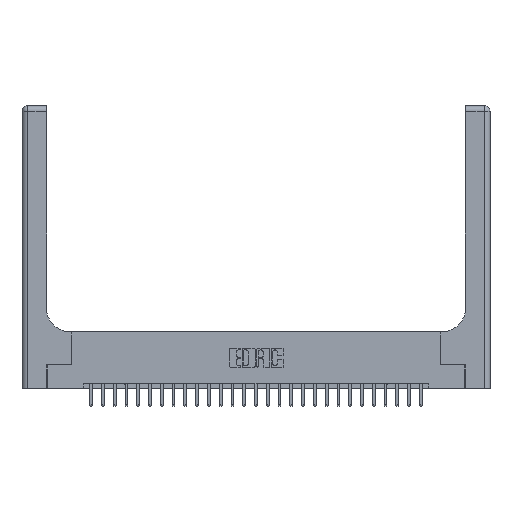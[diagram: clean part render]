
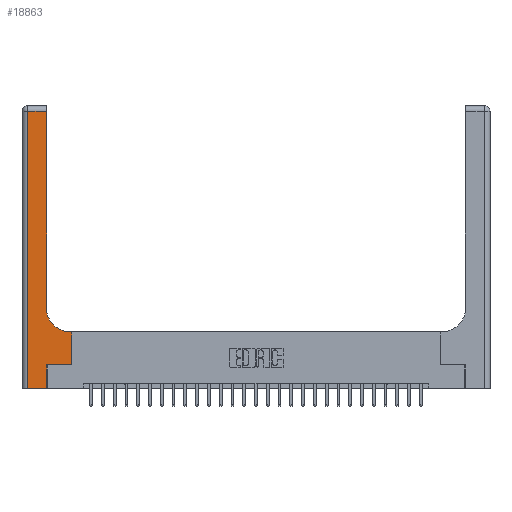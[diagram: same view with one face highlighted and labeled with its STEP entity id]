
A CAD part, top view. The second image highlights one B-rep face of the part: STEP entity #18863.
In plain terms, the highlighted planar face has unit normal (0, 0, 1).
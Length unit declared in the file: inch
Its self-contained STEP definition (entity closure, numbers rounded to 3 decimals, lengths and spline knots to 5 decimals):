
#50 = VERTEX_POINT ( 'NONE', #14233 ) ;
#340 = VERTEX_POINT ( 'NONE', #12329 ) ;
#403 = PLANE ( 'NONE',  #8619 ) ;
#505 = CARTESIAN_POINT ( 'NONE',  ( 0.51, 0.6, 0.37 ) ) ;
#557 = CARTESIAN_POINT ( 'NONE',  ( 0.528, 0.25, 0.37 ) ) ;
#688 = LINE ( 'NONE', #557, #17338 ) ;
#1341 = DIRECTION ( 'NONE',  ( 0., -1., 0. ) ) ;
#1430 = LINE ( 'NONE', #13756, #6898 ) ;
#2548 = DIRECTION ( 'NONE',  ( -1., 0., 0. ) ) ;
#2902 = ORIENTED_EDGE ( 'NONE', *, *, #24737, .T. ) ;
#2943 = EDGE_CURVE ( 'NONE', #15445, #6280, #25921, .T. ) ;
#3306 = EDGE_CURVE ( 'NONE', #50, #6949, #1430, .T. ) ;
#3812 = CARTESIAN_POINT ( 'NONE',  ( 0., 0., 0.37 ) ) ;
#3834 = VECTOR ( 'NONE', #21688, 39.37008 ) ;
#4189 = DIRECTION ( 'NONE',  ( 1., 0., 0. ) ) ;
#4561 = CARTESIAN_POINT ( 'NONE',  ( 0.265, 0.25, 0.37 ) ) ;
#4729 = CARTESIAN_POINT ( 'NONE',  ( 0.528, 0.25, 0.37 ) ) ;
#5106 = EDGE_CURVE ( 'NONE', #21176, #15445, #7725, .T. ) ;
#6278 = DIRECTION ( 'NONE',  ( 0., 0., -1. ) ) ;
#6280 = VERTEX_POINT ( 'NONE', #11537 ) ;
#6291 = CIRCLE ( 'NONE', #9298, 0.25 ) ;
#6699 = ORIENTED_EDGE ( 'NONE', *, *, #5106, .T. ) ;
#6898 = VECTOR ( 'NONE', #7549, 39.37008 ) ;
#6949 = VERTEX_POINT ( 'NONE', #505 ) ;
#7365 = CARTESIAN_POINT ( 'NONE',  ( 0.265, 0., 0.37 ) ) ;
#7463 = CARTESIAN_POINT ( 'NONE',  ( 0., 2.94, 0.37 ) ) ;
#7501 = EDGE_CURVE ( 'NONE', #340, #9209, #17818, .T. ) ;
#7549 = DIRECTION ( 'NONE',  ( -1., 0., 0. ) ) ;
#7725 = LINE ( 'NONE', #19927, #19897 ) ;
#7945 = ORIENTED_EDGE ( 'NONE', *, *, #13240, .T. ) ;
#8368 = ORIENTED_EDGE ( 'NONE', *, *, #14113, .T. ) ;
#8572 = CARTESIAN_POINT ( 'NONE',  ( 0., 3., 0.37 ) ) ;
#8619 = AXIS2_PLACEMENT_3D ( 'NONE', #8572, #6278, #2548 ) ;
#8847 = VECTOR ( 'NONE', #1341, 39.37008 ) ;
#9209 = VERTEX_POINT ( 'NONE', #4561 ) ;
#9298 = AXIS2_PLACEMENT_3D ( 'NONE', #22425, #16543, #4189 ) ;
#9631 = EDGE_LOOP ( 'NONE', ( #6699, #22606, #20917, #18238, #24569, #7945, #2902, #23261, #8368 ) ) ;
#9702 = DIRECTION ( 'NONE',  ( 1., 0., 0. ) ) ;
#9723 = EDGE_CURVE ( 'NONE', #6280, #15460, #14806, .T. ) ;
#10601 = DIRECTION ( 'NONE',  ( 0., 1., 0. ) ) ;
#11537 = CARTESIAN_POINT ( 'NONE',  ( 0.06, 2.94, 0.37 ) ) ;
#11619 = VECTOR ( 'NONE', #19183, 39.37008 ) ;
#12329 = CARTESIAN_POINT ( 'NONE',  ( 0.265, 0., 0.37 ) ) ;
#12386 = VERTEX_POINT ( 'NONE', #4729 ) ;
#13240 = EDGE_CURVE ( 'NONE', #9209, #12386, #19283, .T. ) ;
#13669 = CARTESIAN_POINT ( 'NONE',  ( 0.06, 3., 0.37 ) ) ;
#13756 = CARTESIAN_POINT ( 'NONE',  ( 0.26, 0.6, 0.37 ) ) ;
#14113 = EDGE_CURVE ( 'NONE', #6949, #21176, #6291, .T. ) ;
#14233 = CARTESIAN_POINT ( 'NONE',  ( 0.528, 0.6, 0.37 ) ) ;
#14250 = CARTESIAN_POINT ( 'NONE',  ( 0.26, 0.85, 0.37 ) ) ;
#14806 = LINE ( 'NONE', #13669, #8847 ) ;
#15067 = CARTESIAN_POINT ( 'NONE',  ( 0.06, 0., 0.37 ) ) ;
#15215 = EDGE_CURVE ( 'NONE', #15460, #340, #23785, .T. ) ;
#15445 = VERTEX_POINT ( 'NONE', #17329 ) ;
#15460 = VERTEX_POINT ( 'NONE', #15067 ) ;
#16543 = DIRECTION ( 'NONE',  ( 0., 0., -1. ) ) ;
#17136 = CARTESIAN_POINT ( 'NONE',  ( 0.265, 0.25, 0.37 ) ) ;
#17137 = FACE_OUTER_BOUND ( 'NONE', #9631, .T. ) ;
#17329 = CARTESIAN_POINT ( 'NONE',  ( 0.26, 2.94, 0.37 ) ) ;
#17338 = VECTOR ( 'NONE', #10601, 39.37008 ) ;
#17818 = LINE ( 'NONE', #7365, #3834 ) ;
#18209 = DIRECTION ( 'NONE',  ( 0., 1., 0. ) ) ;
#18238 = ORIENTED_EDGE ( 'NONE', *, *, #15215, .T. ) ;
#18863 = ADVANCED_FACE ( 'NONE', ( #17137 ), #403, .F. ) ;
#19183 = DIRECTION ( 'NONE',  ( -1., 0., 0. ) ) ;
#19283 = LINE ( 'NONE', #17136, #20855 ) ;
#19897 = VECTOR ( 'NONE', #18209, 39.37008 ) ;
#19927 = CARTESIAN_POINT ( 'NONE',  ( 0.26, 3., 0.37 ) ) ;
#20021 = VECTOR ( 'NONE', #9702, 39.37008 ) ;
#20855 = VECTOR ( 'NONE', #21005, 39.37008 ) ;
#20917 = ORIENTED_EDGE ( 'NONE', *, *, #9723, .T. ) ;
#21005 = DIRECTION ( 'NONE',  ( 1., 0., 0. ) ) ;
#21176 = VERTEX_POINT ( 'NONE', #14250 ) ;
#21688 = DIRECTION ( 'NONE',  ( 0., 1., 0. ) ) ;
#22425 = CARTESIAN_POINT ( 'NONE',  ( 0.51, 0.85, 0.37 ) ) ;
#22606 = ORIENTED_EDGE ( 'NONE', *, *, #2943, .T. ) ;
#23261 = ORIENTED_EDGE ( 'NONE', *, *, #3306, .T. ) ;
#23785 = LINE ( 'NONE', #3812, #20021 ) ;
#24569 = ORIENTED_EDGE ( 'NONE', *, *, #7501, .T. ) ;
#24737 = EDGE_CURVE ( 'NONE', #12386, #50, #688, .T. ) ;
#25921 = LINE ( 'NONE', #7463, #11619 ) ;
